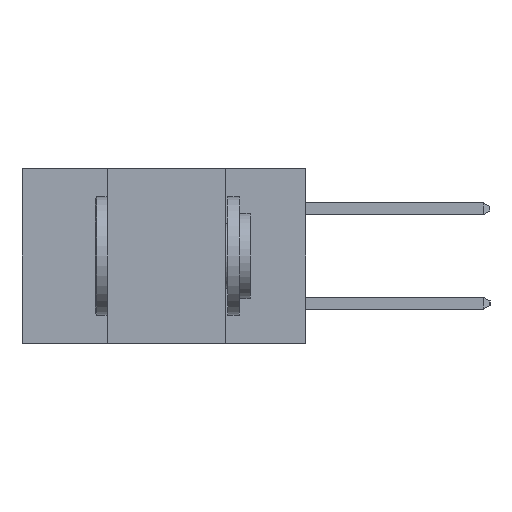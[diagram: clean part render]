
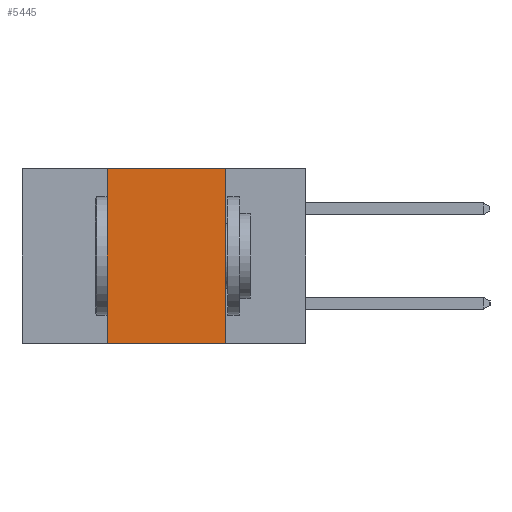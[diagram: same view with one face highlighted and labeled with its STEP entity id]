
A CAD part, left-side view. The second image highlights one B-rep face of the part: STEP entity #5445.
In plain terms, the highlighted planar face has unit normal (-1, 0, 0).
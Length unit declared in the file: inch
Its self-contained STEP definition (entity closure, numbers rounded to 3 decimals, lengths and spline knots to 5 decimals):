
#18 = CARTESIAN_POINT ( 'NONE',  ( 0., 0.17, 0. ) ) ;
#275 = VERTEX_POINT ( 'NONE', #3150 ) ;
#368 = CARTESIAN_POINT ( 'NONE',  ( 0., 0.17, -0.37 ) ) ;
#499 = CARTESIAN_POINT ( 'NONE',  ( 0., 0.42, -0.37 ) ) ;
#574 = EDGE_CURVE ( 'NONE', #5498, #10513, #929, .T. ) ;
#579 = EDGE_CURVE ( 'NONE', #275, #5498, #1901, .T. ) ;
#606 = VECTOR ( 'NONE', #11232, 39.37008 ) ;
#803 = ORIENTED_EDGE ( 'NONE', *, *, #6959, .F. ) ;
#929 = LINE ( 'NONE', #368, #5862 ) ;
#1901 = LINE ( 'NONE', #3617, #606 ) ;
#2012 = LINE ( 'NONE', #499, #7196 ) ;
#3043 = CARTESIAN_POINT ( 'NONE',  ( 0., 0.6, 0. ) ) ;
#3150 = CARTESIAN_POINT ( 'NONE',  ( 0., 0.42, 0. ) ) ;
#3617 = CARTESIAN_POINT ( 'NONE',  ( 0., 0.6, 0. ) ) ;
#3628 = AXIS2_PLACEMENT_3D ( 'NONE', #3043, #9746, #4028 ) ;
#4028 = DIRECTION ( 'NONE',  ( 0., 0., -1. ) ) ;
#4765 = EDGE_LOOP ( 'NONE', ( #9973, #7848, #803, #9323 ) ) ;
#5445 = ADVANCED_FACE ( 'NONE', ( #6637 ), #11086, .F. ) ;
#5498 = VERTEX_POINT ( 'NONE', #18 ) ;
#5862 = VECTOR ( 'NONE', #6667, 39.37008 ) ;
#6095 = DIRECTION ( 'NONE',  ( 0., -1., 0. ) ) ;
#6637 = FACE_OUTER_BOUND ( 'NONE', #4765, .T. ) ;
#6667 = DIRECTION ( 'NONE',  ( 0., 0., -1. ) ) ;
#6784 = EDGE_CURVE ( 'NONE', #9505, #10513, #7650, .T. ) ;
#6816 = CARTESIAN_POINT ( 'NONE',  ( 0., 0.42, -0.37 ) ) ;
#6959 = EDGE_CURVE ( 'NONE', #9505, #275, #2012, .T. ) ;
#7196 = VECTOR ( 'NONE', #7391, 39.37008 ) ;
#7391 = DIRECTION ( 'NONE',  ( 0., 0., 1. ) ) ;
#7650 = LINE ( 'NONE', #11651, #7944 ) ;
#7848 = ORIENTED_EDGE ( 'NONE', *, *, #579, .F. ) ;
#7944 = VECTOR ( 'NONE', #6095, 39.37008 ) ;
#8144 = CARTESIAN_POINT ( 'NONE',  ( 0., 0.17, -0.37 ) ) ;
#9323 = ORIENTED_EDGE ( 'NONE', *, *, #6784, .T. ) ;
#9505 = VERTEX_POINT ( 'NONE', #6816 ) ;
#9746 = DIRECTION ( 'NONE',  ( 1., 0., 0. ) ) ;
#9973 = ORIENTED_EDGE ( 'NONE', *, *, #574, .F. ) ;
#10513 = VERTEX_POINT ( 'NONE', #8144 ) ;
#11086 = PLANE ( 'NONE',  #3628 ) ;
#11232 = DIRECTION ( 'NONE',  ( 0., -1., 0. ) ) ;
#11651 = CARTESIAN_POINT ( 'NONE',  ( 0., 0.6, -0.37 ) ) ;
